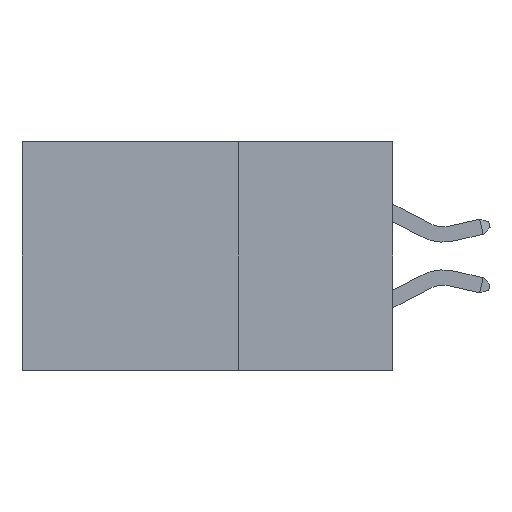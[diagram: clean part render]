
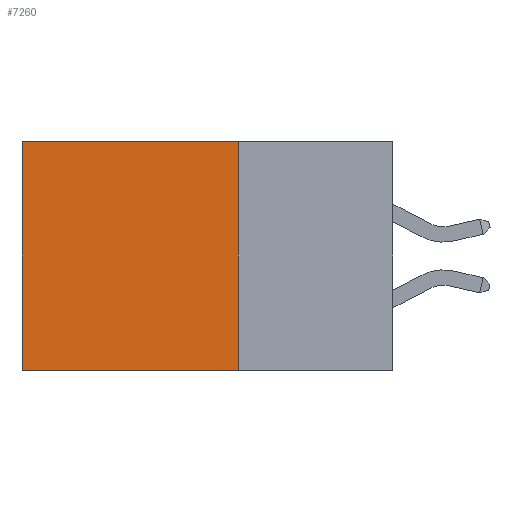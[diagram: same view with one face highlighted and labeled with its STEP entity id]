
A CAD part, left-side view. The second image highlights one B-rep face of the part: STEP entity #7260.
In plain terms, the highlighted planar face has unit normal (-1, 0, 0).
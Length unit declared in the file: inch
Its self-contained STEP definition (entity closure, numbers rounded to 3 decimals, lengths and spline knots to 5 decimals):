
#280 = CARTESIAN_POINT ( 'NONE',  ( 0.2875, 0.6, 0. ) ) ;
#548 = VERTEX_POINT ( 'NONE', #1450 ) ;
#736 = AXIS2_PLACEMENT_3D ( 'NONE', #4935, #10503, #5809 ) ;
#760 = ORIENTED_EDGE ( 'NONE', *, *, #9412, .F. ) ;
#1136 = EDGE_LOOP ( 'NONE', ( #7463, #760, #7713, #9814 ) ) ;
#1142 = VERTEX_POINT ( 'NONE', #4454 ) ;
#1229 = PLANE ( 'NONE',  #736 ) ;
#1313 = CARTESIAN_POINT ( 'NONE',  ( 0.2875, 0.6, 0. ) ) ;
#1450 = CARTESIAN_POINT ( 'NONE',  ( 0.2875, 0.6, -0.37 ) ) ;
#1606 = VECTOR ( 'NONE', #8884, 39.37008 ) ;
#2503 = VECTOR ( 'NONE', #8659, 39.37008 ) ;
#3061 = LINE ( 'NONE', #7170, #2503 ) ;
#3403 = EDGE_CURVE ( 'NONE', #5640, #1142, #4281, .T. ) ;
#4006 = FACE_OUTER_BOUND ( 'NONE', #1136, .T. ) ;
#4281 = LINE ( 'NONE', #5760, #10189 ) ;
#4344 = LINE ( 'NONE', #280, #1606 ) ;
#4454 = CARTESIAN_POINT ( 'NONE',  ( 0.2875, 0.25, -0.37 ) ) ;
#4461 = DIRECTION ( 'NONE',  ( 0., 1., 0. ) ) ;
#4930 = CARTESIAN_POINT ( 'NONE',  ( 0.2875, 0.25, 0. ) ) ;
#4935 = CARTESIAN_POINT ( 'NONE',  ( 0.2875, 0.25, 0. ) ) ;
#5640 = VERTEX_POINT ( 'NONE', #4930 ) ;
#5760 = CARTESIAN_POINT ( 'NONE',  ( 0.2875, 0.25, 0. ) ) ;
#5809 = DIRECTION ( 'NONE',  ( 0., 0., -1. ) ) ;
#5999 = DIRECTION ( 'NONE',  ( 0., 0., -1. ) ) ;
#7168 = LINE ( 'NONE', #8453, #10838 ) ;
#7170 = CARTESIAN_POINT ( 'NONE',  ( 0.2875, 0.25, -0.37 ) ) ;
#7260 = ADVANCED_FACE ( 'NONE', ( #4006 ), #1229, .F. ) ;
#7463 = ORIENTED_EDGE ( 'NONE', *, *, #9054, .T. ) ;
#7713 = ORIENTED_EDGE ( 'NONE', *, *, #3403, .F. ) ;
#8453 = CARTESIAN_POINT ( 'NONE',  ( 0.2875, 0.25, 0. ) ) ;
#8659 = DIRECTION ( 'NONE',  ( 0., 1., 0. ) ) ;
#8884 = DIRECTION ( 'NONE',  ( 0., 0., -1. ) ) ;
#9054 = EDGE_CURVE ( 'NONE', #10233, #548, #4344, .T. ) ;
#9316 = EDGE_CURVE ( 'NONE', #5640, #10233, #7168, .T. ) ;
#9412 = EDGE_CURVE ( 'NONE', #1142, #548, #3061, .T. ) ;
#9814 = ORIENTED_EDGE ( 'NONE', *, *, #9316, .T. ) ;
#10189 = VECTOR ( 'NONE', #5999, 39.37008 ) ;
#10233 = VERTEX_POINT ( 'NONE', #1313 ) ;
#10503 = DIRECTION ( 'NONE',  ( 1., 0., 0. ) ) ;
#10838 = VECTOR ( 'NONE', #4461, 39.37008 ) ;
